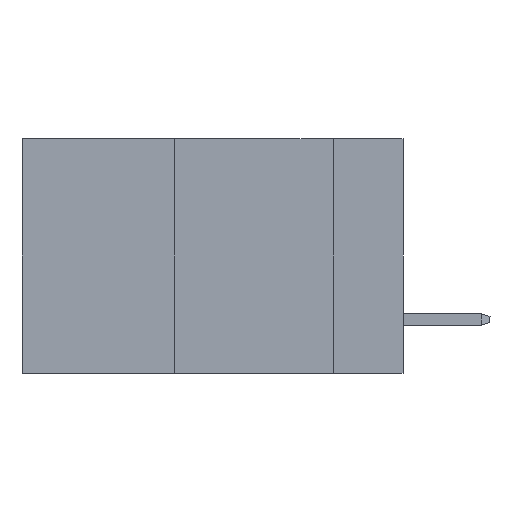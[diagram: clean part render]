
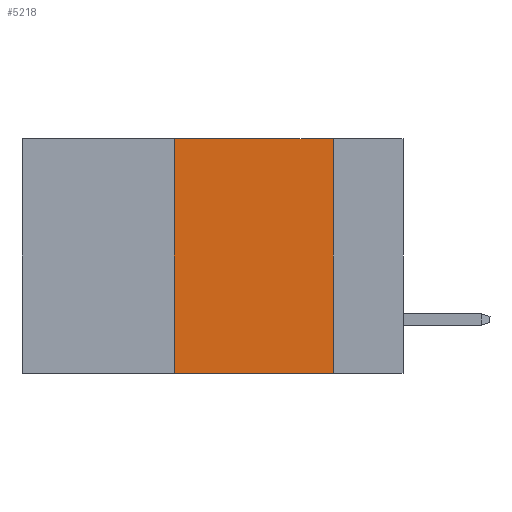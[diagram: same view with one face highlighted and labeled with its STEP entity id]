
A CAD part, left-side view. The second image highlights one B-rep face of the part: STEP entity #5218.
In plain terms, the highlighted planar face has unit normal (-1, 0, 0).
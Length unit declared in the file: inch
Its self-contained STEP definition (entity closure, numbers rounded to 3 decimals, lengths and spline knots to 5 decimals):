
#601 = FACE_OUTER_BOUND ( 'NONE', #16462, .T. ) ;
#648 = CARTESIAN_POINT ( 'NONE',  ( 0., 0.11, 0. ) ) ;
#715 = EDGE_CURVE ( 'NONE', #3506, #16777, #2136, .T. ) ;
#751 = DIRECTION ( 'NONE',  ( 0., -1., 0. ) ) ;
#1007 = EDGE_CURVE ( 'NONE', #15277, #16777, #15031, .T. ) ;
#2136 = LINE ( 'NONE', #12591, #13710 ) ;
#2407 = CARTESIAN_POINT ( 'NONE',  ( 0., 0.6, 0. ) ) ;
#3481 = CARTESIAN_POINT ( 'NONE',  ( 0., 0.11, -0.37 ) ) ;
#3506 = VERTEX_POINT ( 'NONE', #9976 ) ;
#4545 = DIRECTION ( 'NONE',  ( 1., 0., 0. ) ) ;
#4941 = AXIS2_PLACEMENT_3D ( 'NONE', #11059, #4545, #14981 ) ;
#5055 = DIRECTION ( 'NONE',  ( 0., -1., 0. ) ) ;
#5218 = ADVANCED_FACE ( 'NONE', ( #601 ), #14648, .F. ) ;
#5724 = ORIENTED_EDGE ( 'NONE', *, *, #15034, .F. ) ;
#6190 = CARTESIAN_POINT ( 'NONE',  ( 0., 0.36, 0. ) ) ;
#8375 = EDGE_CURVE ( 'NONE', #12206, #15277, #12932, .T. ) ;
#9976 = CARTESIAN_POINT ( 'NONE',  ( 0., 0.36, -0.37 ) ) ;
#10063 = DIRECTION ( 'NONE',  ( 0., 0., 1. ) ) ;
#10574 = ORIENTED_EDGE ( 'NONE', *, *, #8375, .F. ) ;
#10854 = VECTOR ( 'NONE', #10063, 39.37008 ) ;
#11059 = CARTESIAN_POINT ( 'NONE',  ( 0., 0.6, 0. ) ) ;
#11178 = DIRECTION ( 'NONE',  ( 0., 0., -1. ) ) ;
#11236 = CARTESIAN_POINT ( 'NONE',  ( 0., 0.11, 0. ) ) ;
#12206 = VERTEX_POINT ( 'NONE', #6190 ) ;
#12540 = ORIENTED_EDGE ( 'NONE', *, *, #1007, .F. ) ;
#12591 = CARTESIAN_POINT ( 'NONE',  ( 0., 0.6, -0.37 ) ) ;
#12932 = LINE ( 'NONE', #2407, #13648 ) ;
#13648 = VECTOR ( 'NONE', #5055, 39.37008 ) ;
#13710 = VECTOR ( 'NONE', #751, 39.37008 ) ;
#13981 = VECTOR ( 'NONE', #11178, 39.37008 ) ;
#14648 = PLANE ( 'NONE',  #4941 ) ;
#14981 = DIRECTION ( 'NONE',  ( 0., 0., -1. ) ) ;
#15031 = LINE ( 'NONE', #648, #13981 ) ;
#15034 = EDGE_CURVE ( 'NONE', #3506, #12206, #15104, .T. ) ;
#15104 = LINE ( 'NONE', #16671, #10854 ) ;
#15277 = VERTEX_POINT ( 'NONE', #11236 ) ;
#16223 = ORIENTED_EDGE ( 'NONE', *, *, #715, .T. ) ;
#16462 = EDGE_LOOP ( 'NONE', ( #12540, #10574, #5724, #16223 ) ) ;
#16671 = CARTESIAN_POINT ( 'NONE',  ( 0., 0.36, 0. ) ) ;
#16777 = VERTEX_POINT ( 'NONE', #3481 ) ;
